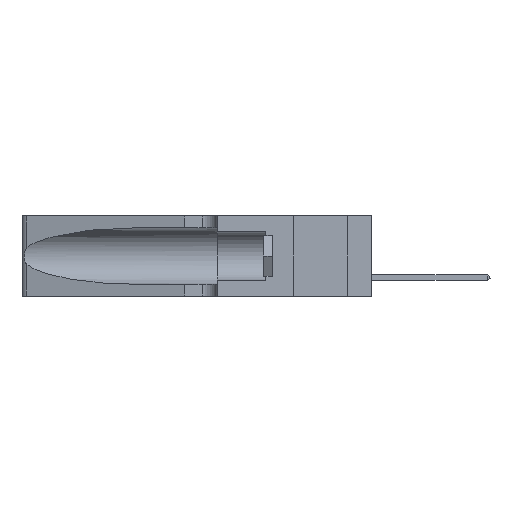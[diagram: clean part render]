
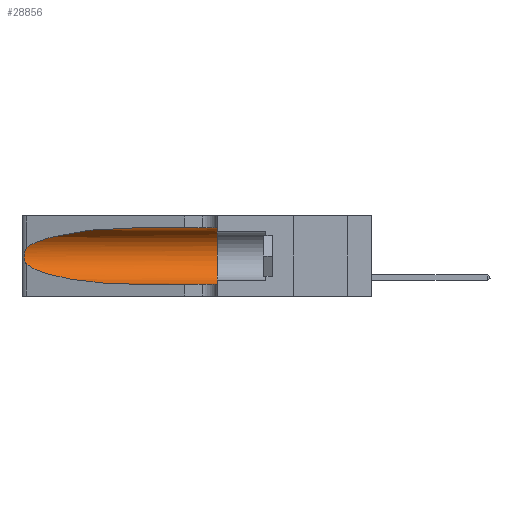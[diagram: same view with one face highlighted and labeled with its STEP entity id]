
A CAD part, left-side view. The second image highlights one B-rep face of the part: STEP entity #28856.
In plain terms, the highlighted cylindrical face has radius 3.308 mm (diameter 6.617 mm), a partial arc.
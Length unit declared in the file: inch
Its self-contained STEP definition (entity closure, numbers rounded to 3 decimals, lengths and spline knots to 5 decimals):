
#279 = EDGE_CURVE ( 'NONE', #15581, #7552, #6661, .T. ) ;
#860 = CARTESIAN_POINT ( 'NONE',  ( 0.25639, 1.23184, 0.21858 ) ) ;
#938 = ORIENTED_EDGE ( 'NONE', *, *, #2107, .T. ) ;
#1587 = CARTESIAN_POINT ( 'NONE',  ( 0.25555, 1.22994, 0.2215 ) ) ;
#2107 = EDGE_CURVE ( 'NONE', #28356, #15581, #30528, .T. ) ;
#2598 = CARTESIAN_POINT ( 'NONE',  ( 0.18966, 0.96281, 0.05475 ) ) ;
#4578 = AXIS2_PLACEMENT_3D ( 'NONE', #6463, #9288, #15565 ) ;
#5098 =( BOUNDED_CURVE ( )  B_SPLINE_CURVE ( 3, ( #20622, #24957, #2598, #21958 ),
 .UNSPECIFIED., .F., .T. ) 
 B_SPLINE_CURVE_WITH_KNOTS ( ( 4, 4 ),
 ( 3.44316, 4.71239 ),
 .UNSPECIFIED. ) 
 CURVE ( )  GEOMETRIC_REPRESENTATION_ITEM ( )  RATIONAL_B_SPLINE_CURVE ( ( 1., 0.87, 0.87, 1. ) ) 
 REPRESENTATION_ITEM ( '' )  );
#5987 = CARTESIAN_POINT ( 'NONE',  ( 0.18966, 0.96281, 0.31525 ) ) ;
#6123 = VERTEX_POINT ( 'NONE', #21401 ) ;
#6463 = CARTESIAN_POINT ( 'NONE',  ( 0.1305, 0.35, 0.185 ) ) ;
#6661 = B_SPLINE_CURVE_WITH_KNOTS ( 'NONE', 3,
 ( #12456, #1587, #860, #7719, #10102, #35361, #21360, #15621, #32177, #7759, #30329, #11404, #8382, #22445 ),
 .UNSPECIFIED., .F., .F.,
 ( 4, 2, 2, 2, 2, 2, 4 ),
 ( 0., 0.00027, 0.00053, 0.00107, 0.0016, 0.00187, 0.00214 ),
 .UNSPECIFIED. ) ;
#6936 = ORIENTED_EDGE ( 'NONE', *, *, #26874, .F. ) ;
#7552 = VERTEX_POINT ( 'NONE', #30234 ) ;
#7719 = CARTESIAN_POINT ( 'NONE',  ( 0.25787, 1.23484, 0.2124 ) ) ;
#7759 = CARTESIAN_POINT ( 'NONE',  ( 0.25856, 1.23593, 0.16098 ) ) ;
#7769 = CARTESIAN_POINT ( 'NONE',  ( 0.1305, 0.72297, 0.31525 ) ) ;
#8382 = CARTESIAN_POINT ( 'NONE',  ( 0.25555, 1.22993, 0.14849 ) ) ;
#8550 = EDGE_CURVE ( 'NONE', #6123, #16542, #27878, .T. ) ;
#9288 = DIRECTION ( 'NONE',  ( 0., 1., 0. ) ) ;
#10102 = CARTESIAN_POINT ( 'NONE',  ( 0.25854, 1.2359, 0.20912 ) ) ;
#11404 = CARTESIAN_POINT ( 'NONE',  ( 0.25639, 1.23186, 0.15144 ) ) ;
#12456 = CARTESIAN_POINT ( 'NONE',  ( 0.25487, 1.22718, 0.22369 ) ) ;
#12985 = EDGE_CURVE ( 'NONE', #16109, #16542, #18803, .T. ) ;
#13129 = ORIENTED_EDGE ( 'NONE', *, *, #21821, .T. ) ;
#13152 = CARTESIAN_POINT ( 'NONE',  ( 0.1305, 0.72297, 0.31525 ) ) ;
#14526 = CARTESIAN_POINT ( 'NONE',  ( 0.2373, 1.15595, 0.28018 ) ) ;
#14537 = AXIS2_PLACEMENT_3D ( 'NONE', #26492, #23386, #23510 ) ;
#14703 = ORIENTED_EDGE ( 'NONE', *, *, #12985, .F. ) ;
#15565 = DIRECTION ( 'NONE',  ( 0., 0., 1. ) ) ;
#15581 = VERTEX_POINT ( 'NONE', #33854 ) ;
#15621 = CARTESIAN_POINT ( 'NONE',  ( 0.26075, 1.23896, 0.178 ) ) ;
#16109 = VERTEX_POINT ( 'NONE', #30512 ) ;
#16542 = VERTEX_POINT ( 'NONE', #23231 ) ;
#18803 = CIRCLE ( 'NONE', #4578, 0.13025 ) ;
#20622 = CARTESIAN_POINT ( 'NONE',  ( 0.25487, 1.22718, 0.14631 ) ) ;
#21084 = DIRECTION ( 'NONE',  ( 0., -1., 0. ) ) ;
#21360 = CARTESIAN_POINT ( 'NONE',  ( 0.26075, 1.23896, 0.19203 ) ) ;
#21401 = CARTESIAN_POINT ( 'NONE',  ( 0.1305, 0.72297, 0.05475 ) ) ;
#21821 = EDGE_CURVE ( 'NONE', #7552, #6123, #5098, .T. ) ;
#21824 = CYLINDRICAL_SURFACE ( 'NONE', #14537, 0.13025 ) ;
#21958 = CARTESIAN_POINT ( 'NONE',  ( 0.1305, 0.72297, 0.05475 ) ) ;
#22445 = CARTESIAN_POINT ( 'NONE',  ( 0.25487, 1.22718, 0.14631 ) ) ;
#23231 = CARTESIAN_POINT ( 'NONE',  ( 0.1305, 0.35, 0.05475 ) ) ;
#23386 = DIRECTION ( 'NONE',  ( 0., -1., 0. ) ) ;
#23510 = DIRECTION ( 'NONE',  ( 0., 0., -1. ) ) ;
#24957 = CARTESIAN_POINT ( 'NONE',  ( 0.2373, 1.15595, 0.08982 ) ) ;
#25494 = CARTESIAN_POINT ( 'NONE',  ( 0.1305, 1.61858, 0.31525 ) ) ;
#25518 = LINE ( 'NONE', #25494, #31623 ) ;
#26492 = CARTESIAN_POINT ( 'NONE',  ( 0.1305, 1.61858, 0.185 ) ) ;
#26874 = EDGE_CURVE ( 'NONE', #28356, #16109, #25518, .T. ) ;
#27736 = ORIENTED_EDGE ( 'NONE', *, *, #279, .T. ) ;
#27878 = LINE ( 'NONE', #30049, #31349 ) ;
#28090 = CARTESIAN_POINT ( 'NONE',  ( 0.25487, 1.22718, 0.22369 ) ) ;
#28356 = VERTEX_POINT ( 'NONE', #13152 ) ;
#28361 = FACE_OUTER_BOUND ( 'NONE', #28815, .T. ) ;
#28815 = EDGE_LOOP ( 'NONE', ( #938, #27736, #13129, #33653, #14703, #6936 ) ) ;
#28856 = ADVANCED_FACE ( 'NONE', ( #28361 ), #21824, .F. ) ;
#30049 = CARTESIAN_POINT ( 'NONE',  ( 0.1305, 1.61858, 0.05475 ) ) ;
#30234 = CARTESIAN_POINT ( 'NONE',  ( 0.25487, 1.22718, 0.14631 ) ) ;
#30329 = CARTESIAN_POINT ( 'NONE',  ( 0.25789, 1.23486, 0.15765 ) ) ;
#30512 = CARTESIAN_POINT ( 'NONE',  ( 0.1305, 0.35, 0.31525 ) ) ;
#30528 =( BOUNDED_CURVE ( )  B_SPLINE_CURVE ( 3, ( #7769, #5987, #14526, #28090 ),
 .UNSPECIFIED., .F., .T. ) 
 B_SPLINE_CURVE_WITH_KNOTS ( ( 4, 4 ),
 ( 1.5708, 2.84003 ),
 .UNSPECIFIED. ) 
 CURVE ( )  GEOMETRIC_REPRESENTATION_ITEM ( )  RATIONAL_B_SPLINE_CURVE ( ( 1., 0.87, 0.87, 1. ) ) 
 REPRESENTATION_ITEM ( '' )  );
#30989 = DIRECTION ( 'NONE',  ( 0., -1., 0. ) ) ;
#31349 = VECTOR ( 'NONE', #21084, 39.37008 ) ;
#31623 = VECTOR ( 'NONE', #30989, 39.37008 ) ;
#32177 = CARTESIAN_POINT ( 'NONE',  ( 0.26017, 1.23833, 0.17102 ) ) ;
#33653 = ORIENTED_EDGE ( 'NONE', *, *, #8550, .T. ) ;
#33854 = CARTESIAN_POINT ( 'NONE',  ( 0.25487, 1.22718, 0.22369 ) ) ;
#35361 = CARTESIAN_POINT ( 'NONE',  ( 0.26018, 1.23835, 0.19895 ) ) ;
